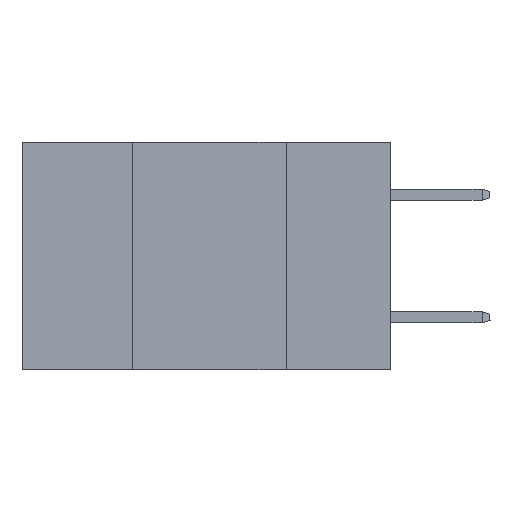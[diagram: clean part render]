
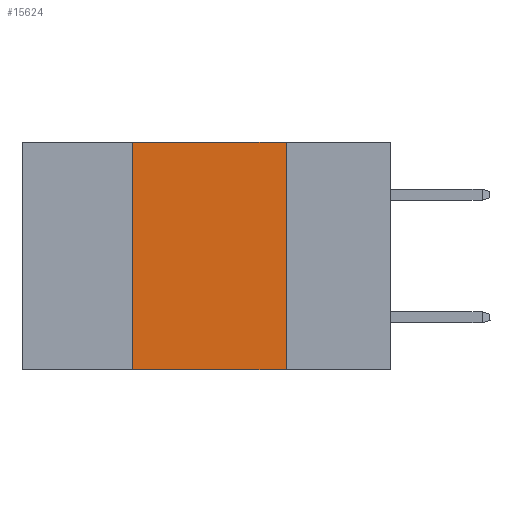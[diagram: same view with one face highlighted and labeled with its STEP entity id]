
A CAD part, left-side view. The second image highlights one B-rep face of the part: STEP entity #15624.
In plain terms, the highlighted planar face has unit normal (-1, 0, 0).
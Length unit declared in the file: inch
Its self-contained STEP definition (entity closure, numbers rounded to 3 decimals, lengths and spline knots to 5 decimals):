
#44 = EDGE_LOOP ( 'NONE', ( #13081, #10268, #2670, #5807 ) ) ;
#543 = AXIS2_PLACEMENT_3D ( 'NONE', #3343, #1877, #14588 ) ;
#813 = EDGE_CURVE ( 'NONE', #18352, #3434, #14579, .T. ) ;
#932 = CARTESIAN_POINT ( 'NONE',  ( 0., 0.17, 0. ) ) ;
#1762 = VECTOR ( 'NONE', #13230, 39.37008 ) ;
#1877 = DIRECTION ( 'NONE',  ( 1., 0., 0. ) ) ;
#2406 = VECTOR ( 'NONE', #15077, 39.37008 ) ;
#2670 = ORIENTED_EDGE ( 'NONE', *, *, #3806, .F. ) ;
#3026 = FACE_OUTER_BOUND ( 'NONE', #44, .T. ) ;
#3343 = CARTESIAN_POINT ( 'NONE',  ( 0., 0.6, 0. ) ) ;
#3434 = VERTEX_POINT ( 'NONE', #14115 ) ;
#3806 = EDGE_CURVE ( 'NONE', #17278, #15047, #5389, .T. ) ;
#4728 = CARTESIAN_POINT ( 'NONE',  ( 0., 0.6, -0.37 ) ) ;
#5216 = VECTOR ( 'NONE', #20810, 39.37008 ) ;
#5389 = LINE ( 'NONE', #9246, #6156 ) ;
#5807 = ORIENTED_EDGE ( 'NONE', *, *, #16746, .T. ) ;
#6156 = VECTOR ( 'NONE', #9041, 39.37008 ) ;
#6660 = LINE ( 'NONE', #13452, #2406 ) ;
#9041 = DIRECTION ( 'NONE',  ( 0., 0., 1. ) ) ;
#9246 = CARTESIAN_POINT ( 'NONE',  ( 0., 0.42, 0. ) ) ;
#10268 = ORIENTED_EDGE ( 'NONE', *, *, #18242, .F. ) ;
#11107 = CARTESIAN_POINT ( 'NONE',  ( 0., 0.42, -0.37 ) ) ;
#13081 = ORIENTED_EDGE ( 'NONE', *, *, #813, .F. ) ;
#13119 = PLANE ( 'NONE',  #543 ) ;
#13230 = DIRECTION ( 'NONE',  ( 0., 0., -1. ) ) ;
#13357 = CARTESIAN_POINT ( 'NONE',  ( 0., 0.42, 0. ) ) ;
#13452 = CARTESIAN_POINT ( 'NONE',  ( 0., 0.6, 0. ) ) ;
#14115 = CARTESIAN_POINT ( 'NONE',  ( 0., 0.17, -0.37 ) ) ;
#14579 = LINE ( 'NONE', #14774, #1762 ) ;
#14588 = DIRECTION ( 'NONE',  ( 0., 0., -1. ) ) ;
#14774 = CARTESIAN_POINT ( 'NONE',  ( 0., 0.17, 0. ) ) ;
#15047 = VERTEX_POINT ( 'NONE', #13357 ) ;
#15077 = DIRECTION ( 'NONE',  ( 0., -1., 0. ) ) ;
#15624 = ADVANCED_FACE ( 'NONE', ( #3026 ), #13119, .F. ) ;
#16746 = EDGE_CURVE ( 'NONE', #17278, #3434, #20799, .T. ) ;
#17278 = VERTEX_POINT ( 'NONE', #11107 ) ;
#18242 = EDGE_CURVE ( 'NONE', #15047, #18352, #6660, .T. ) ;
#18352 = VERTEX_POINT ( 'NONE', #932 ) ;
#20799 = LINE ( 'NONE', #4728, #5216 ) ;
#20810 = DIRECTION ( 'NONE',  ( 0., -1., 0. ) ) ;
